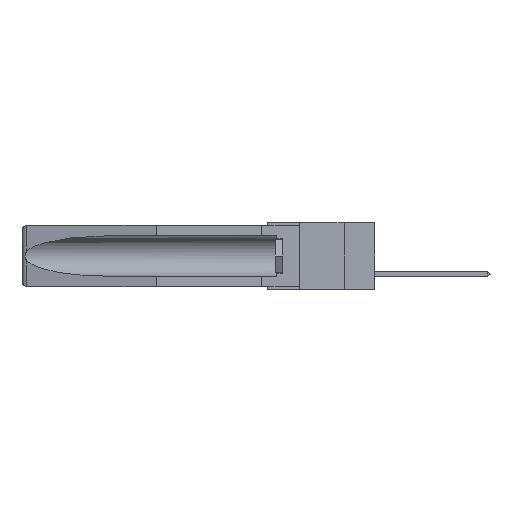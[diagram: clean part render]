
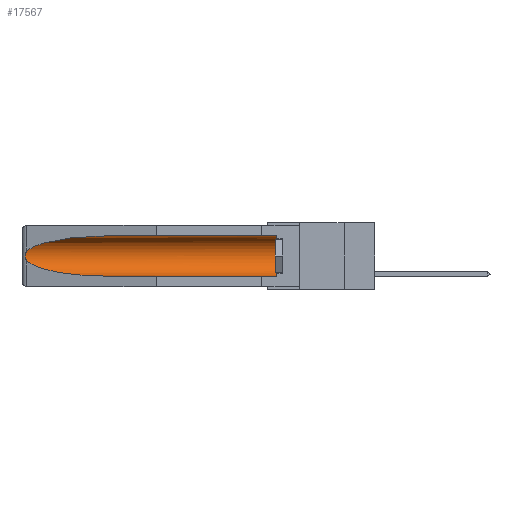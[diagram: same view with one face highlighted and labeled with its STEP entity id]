
A CAD part, left-side view. The second image highlights one B-rep face of the part: STEP entity #17567.
In plain terms, the highlighted cylindrical face has radius 2.857 mm (diameter 5.715 mm), a partial arc.
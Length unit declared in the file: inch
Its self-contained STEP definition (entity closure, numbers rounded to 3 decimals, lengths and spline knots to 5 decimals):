
#130 = ORIENTED_EDGE ( 'NONE', *, *, #18394, .T. ) ;
#271 = DIRECTION ( 'NONE',  ( 0., 1., 0. ) ) ;
#570 = CARTESIAN_POINT ( 'NONE',  ( 0.26537, 1.52718, -0.19328 ) ) ;
#618 = VERTEX_POINT ( 'NONE', #5965 ) ;
#978 = DIRECTION ( 'NONE',  ( 0., 1., 0. ) ) ;
#1134 = CARTESIAN_POINT ( 'NONE',  ( 0.25451, 1.48313, -0.09465 ) ) ;
#1627 = AXIS2_PLACEMENT_3D ( 'NONE', #13370, #13450, #11651 ) ;
#1679 = CARTESIAN_POINT ( 'NONE',  ( 0.26537, 1.52718, -0.19328 ) ) ;
#1812 = CARTESIAN_POINT ( 'NONE',  ( 0.155, -0.30754, -0.284 ) ) ;
#2138 = CARTESIAN_POINT ( 'NONE',  ( 0.155, -0.30754, -0.1715 ) ) ;
#2335 = CARTESIAN_POINT ( 'NONE',  ( 0.2673, 1.5327, -0.16383 ) ) ;
#2517 = B_SPLINE_CURVE_WITH_KNOTS ( 'NONE', 3,
 ( #11857, #4436, #17431, #2335, #6388, #20926, #10064, #11928, #22752, #570 ),
 .UNSPECIFIED., .F., .F.,
 ( 4, 2, 2, 2, 4 ),
 ( 0., 0.00029, 0.00058, 0.00087, 0.00117 ),
 .UNSPECIFIED. ) ;
#2658 = CARTESIAN_POINT ( 'NONE',  ( 0.155, -0.30754, -0.059 ) ) ;
#2894 = EDGE_CURVE ( 'NONE', #8087, #618, #18011, .T. ) ;
#4436 = CARTESIAN_POINT ( 'NONE',  ( 0.26597, 1.52961, -0.15275 ) ) ;
#5182 = CARTESIAN_POINT ( 'NONE',  ( 0.155, 1.07973, -0.284 ) ) ;
#5410 = CARTESIAN_POINT ( 'NONE',  ( 0.25451, 1.48313, -0.24835 ) ) ;
#5550 = CARTESIAN_POINT ( 'NONE',  ( 0.155, 1.07973, -0.059 ) ) ;
#5749 = CARTESIAN_POINT ( 'NONE',  ( 0.155, 0.126, -0.059 ) ) ;
#5965 = CARTESIAN_POINT ( 'NONE',  ( 0.155, 1.07973, -0.284 ) ) ;
#6388 = CARTESIAN_POINT ( 'NONE',  ( 0.2675, 1.53308, -0.16763 ) ) ;
#7246 = EDGE_CURVE ( 'NONE', #23838, #618, #23407, .T. ) ;
#8087 = VERTEX_POINT ( 'NONE', #15252 ) ;
#10064 = CARTESIAN_POINT ( 'NONE',  ( 0.2673, 1.53269, -0.17917 ) ) ;
#10646 = EDGE_LOOP ( 'NONE', ( #16514, #130, #15635, #23074, #16613, #10817 ) ) ;
#10817 = ORIENTED_EDGE ( 'NONE', *, *, #11416, .T. ) ;
#10994 = VERTEX_POINT ( 'NONE', #5550 ) ;
#11416 = EDGE_CURVE ( 'NONE', #19462, #10994, #17228, .T. ) ;
#11651 = DIRECTION ( 'NONE',  ( 0., 0., 1. ) ) ;
#11857 = CARTESIAN_POINT ( 'NONE',  ( 0.26537, 1.52718, -0.14972 ) ) ;
#11928 = CARTESIAN_POINT ( 'NONE',  ( 0.26655, 1.53094, -0.18657 ) ) ;
#12590 = CARTESIAN_POINT ( 'NONE',  ( 0.21114, 1.30732, -0.284 ) ) ;
#13370 = CARTESIAN_POINT ( 'NONE',  ( 0.155, 0.126, -0.1715 ) ) ;
#13404 = EDGE_CURVE ( 'NONE', #10994, #19906, #20836, .T. ) ;
#13450 = DIRECTION ( 'NONE',  ( 0., -1., 0. ) ) ;
#13636 = AXIS2_PLACEMENT_3D ( 'NONE', #2138, #271, #18789 ) ;
#14747 = DIRECTION ( 'NONE',  ( 0., 1., 0. ) ) ;
#14761 = VECTOR ( 'NONE', #14747, 39.37008 ) ;
#15205 = VECTOR ( 'NONE', #978, 39.37008 ) ;
#15252 = CARTESIAN_POINT ( 'NONE',  ( 0.26537, 1.52718, -0.19328 ) ) ;
#15635 = ORIENTED_EDGE ( 'NONE', *, *, #2894, .T. ) ;
#15832 = CARTESIAN_POINT ( 'NONE',  ( 0.155, 1.07973, -0.059 ) ) ;
#16144 = CARTESIAN_POINT ( 'NONE',  ( 0.26537, 1.52718, -0.14972 ) ) ;
#16514 = ORIENTED_EDGE ( 'NONE', *, *, #13404, .T. ) ;
#16613 = ORIENTED_EDGE ( 'NONE', *, *, #17708, .T. ) ;
#16715 = CYLINDRICAL_SURFACE ( 'NONE', #13636, 0.1125 ) ;
#17228 = LINE ( 'NONE', #2658, #15205 ) ;
#17431 = CARTESIAN_POINT ( 'NONE',  ( 0.26654, 1.53092, -0.15636 ) ) ;
#17567 = ADVANCED_FACE ( 'NONE', ( #19888 ), #16715, .F. ) ;
#17708 = EDGE_CURVE ( 'NONE', #23838, #19462, #23307, .T. ) ;
#18011 =( BOUNDED_CURVE ( )  B_SPLINE_CURVE ( 3, ( #1679, #5410, #12590, #5182 ),
 .UNSPECIFIED., .F., .F. ) 
 B_SPLINE_CURVE_WITH_KNOTS ( ( 4, 4 ),
 ( 0.1948, 1.5708 ),
 .UNSPECIFIED. ) 
 CURVE ( )  GEOMETRIC_REPRESENTATION_ITEM ( )  RATIONAL_B_SPLINE_CURVE ( ( 1., 0.848, 0.848, 1. ) ) 
 REPRESENTATION_ITEM ( '' )  );
#18394 = EDGE_CURVE ( 'NONE', #19906, #8087, #2517, .T. ) ;
#18789 = DIRECTION ( 'NONE',  ( 0., 0., 1. ) ) ;
#19462 = VERTEX_POINT ( 'NONE', #5749 ) ;
#19888 = FACE_OUTER_BOUND ( 'NONE', #10646, .T. ) ;
#19906 = VERTEX_POINT ( 'NONE', #16144 ) ;
#20276 = CARTESIAN_POINT ( 'NONE',  ( 0.155, 0.126, -0.284 ) ) ;
#20836 =( BOUNDED_CURVE ( )  B_SPLINE_CURVE ( 3, ( #15832, #21582, #1134, #21415 ),
 .UNSPECIFIED., .F., .F. ) 
 B_SPLINE_CURVE_WITH_KNOTS ( ( 4, 4 ),
 ( 4.71239, 6.08839 ),
 .UNSPECIFIED. ) 
 CURVE ( )  GEOMETRIC_REPRESENTATION_ITEM ( )  RATIONAL_B_SPLINE_CURVE ( ( 1., 0.848, 0.848, 1. ) ) 
 REPRESENTATION_ITEM ( '' )  );
#20926 = CARTESIAN_POINT ( 'NONE',  ( 0.2675, 1.53308, -0.17534 ) ) ;
#21415 = CARTESIAN_POINT ( 'NONE',  ( 0.26537, 1.52718, -0.14972 ) ) ;
#21582 = CARTESIAN_POINT ( 'NONE',  ( 0.21114, 1.30732, -0.059 ) ) ;
#22752 = CARTESIAN_POINT ( 'NONE',  ( 0.26597, 1.5296, -0.19026 ) ) ;
#23074 = ORIENTED_EDGE ( 'NONE', *, *, #7246, .F. ) ;
#23307 = CIRCLE ( 'NONE', #1627, 0.1125 ) ;
#23407 = LINE ( 'NONE', #1812, #14761 ) ;
#23838 = VERTEX_POINT ( 'NONE', #20276 ) ;
